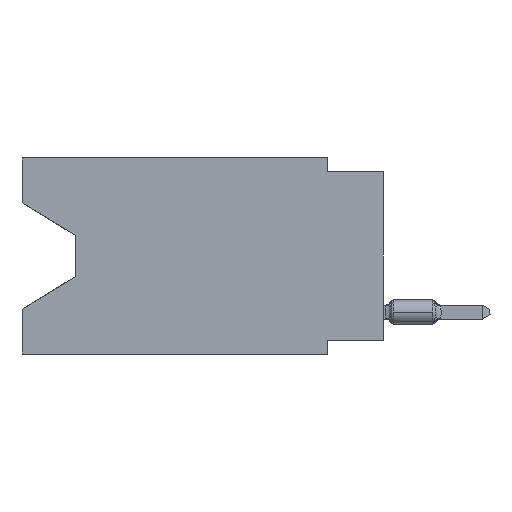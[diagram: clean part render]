
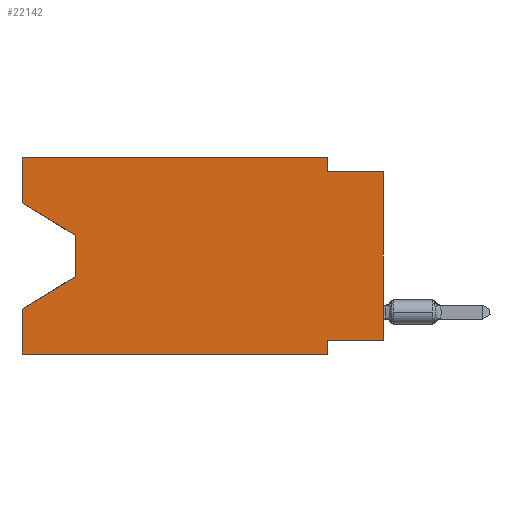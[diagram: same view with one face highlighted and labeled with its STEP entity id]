
A CAD part, left-side view. The second image highlights one B-rep face of the part: STEP entity #22142.
In plain terms, the highlighted planar face has unit normal (-1, 0, 0).
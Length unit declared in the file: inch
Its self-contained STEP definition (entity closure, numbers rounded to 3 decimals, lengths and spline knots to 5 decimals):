
#1131 = VECTOR ( 'NONE', #43221, 39.37008 ) ;
#1315 = VECTOR ( 'NONE', #15655, 39.37008 ) ;
#1429 = VECTOR ( 'NONE', #44214, 39.37008 ) ;
#1787 = EDGE_CURVE ( 'NONE', #48189, #27708, #22861, .T. ) ;
#2738 = CARTESIAN_POINT ( 'NONE',  ( 0., 0.645, 0. ) ) ;
#2757 = DIRECTION ( 'NONE',  ( 1., 0., 0. ) ) ;
#2975 = LINE ( 'NONE', #22295, #7752 ) ;
#3117 = VERTEX_POINT ( 'NONE', #30877 ) ;
#3692 = CARTESIAN_POINT ( 'NONE',  ( 0., 0.1, -0.35 ) ) ;
#3743 = LINE ( 'NONE', #29391, #39164 ) ;
#4198 = EDGE_CURVE ( 'NONE', #3117, #31693, #40388, .T. ) ;
#4311 = ORIENTED_EDGE ( 'NONE', *, *, #17514, .F. ) ;
#4424 = CARTESIAN_POINT ( 'NONE',  ( 0., 0.1, 0. ) ) ;
#4517 = DIRECTION ( 'NONE',  ( 0., 1., 0. ) ) ;
#4624 = CARTESIAN_POINT ( 'NONE',  ( 0., 0.1, 0. ) ) ;
#4648 = CARTESIAN_POINT ( 'NONE',  ( 0., 0.55, -0.138 ) ) ;
#4979 = ORIENTED_EDGE ( 'NONE', *, *, #4198, .F. ) ;
#5315 = CARTESIAN_POINT ( 'NONE',  ( 0., 0.1, -0.325 ) ) ;
#5489 = CARTESIAN_POINT ( 'NONE',  ( 0., 0., 0. ) ) ;
#5548 = CARTESIAN_POINT ( 'NONE',  ( 0., 0.645, -0.08025 ) ) ;
#6111 = VERTEX_POINT ( 'NONE', #2738 ) ;
#6238 = VERTEX_POINT ( 'NONE', #3692 ) ;
#6600 = VECTOR ( 'NONE', #21894, 39.37008 ) ;
#6947 = DIRECTION ( 'NONE',  ( 0., -1., 0. ) ) ;
#6990 = CARTESIAN_POINT ( 'NONE',  ( 0., 0., -0.025 ) ) ;
#7143 = DIRECTION ( 'NONE',  ( 0., 0., 1. ) ) ;
#7667 = CARTESIAN_POINT ( 'NONE',  ( 0., 0.645, 0. ) ) ;
#7752 = VECTOR ( 'NONE', #7143, 39.37008 ) ;
#8032 = ORIENTED_EDGE ( 'NONE', *, *, #1787, .F. ) ;
#8071 = EDGE_CURVE ( 'NONE', #24032, #3117, #37596, .T. ) ;
#10080 = LINE ( 'NONE', #39348, #1131 ) ;
#10835 = DIRECTION ( 'NONE',  ( 0., -1., 0. ) ) ;
#12255 = VERTEX_POINT ( 'NONE', #25113 ) ;
#13143 = ORIENTED_EDGE ( 'NONE', *, *, #36970, .T. ) ;
#13161 = EDGE_CURVE ( 'NONE', #6111, #24032, #3743, .T. ) ;
#14083 = DIRECTION ( 'NONE',  ( 0., 0., -1. ) ) ;
#14225 = ORIENTED_EDGE ( 'NONE', *, *, #33411, .F. ) ;
#14714 = VECTOR ( 'NONE', #14083, 39.37008 ) ;
#14769 = EDGE_CURVE ( 'NONE', #48069, #12255, #40587, .T. ) ;
#15655 = DIRECTION ( 'NONE',  ( 0., 0., -1. ) ) ;
#17514 = EDGE_CURVE ( 'NONE', #40342, #6111, #2975, .T. ) ;
#17635 = DIRECTION ( 'NONE',  ( 0., 0., -1. ) ) ;
#18287 = EDGE_CURVE ( 'NONE', #35943, #12255, #40585, .T. ) ;
#20772 = EDGE_CURVE ( 'NONE', #39972, #48069, #21679, .T. ) ;
#21679 = LINE ( 'NONE', #26050, #43831 ) ;
#21894 = DIRECTION ( 'NONE',  ( 0., -1., 0. ) ) ;
#22142 = ADVANCED_FACE ( 'NONE', ( #28397 ), #47104, .F. ) ;
#22156 = EDGE_CURVE ( 'NONE', #40342, #39972, #10080, .T. ) ;
#22295 = CARTESIAN_POINT ( 'NONE',  ( 0., 0.645, 0. ) ) ;
#22577 = CARTESIAN_POINT ( 'NONE',  ( 0., 0.645, -0.35 ) ) ;
#22861 = LINE ( 'NONE', #30881, #37675 ) ;
#22961 = VECTOR ( 'NONE', #6947, 39.37008 ) ;
#24032 = VERTEX_POINT ( 'NONE', #4624 ) ;
#24141 = ORIENTED_EDGE ( 'NONE', *, *, #13161, .F. ) ;
#25113 = CARTESIAN_POINT ( 'NONE',  ( 0., 0.645, -0.26975 ) ) ;
#26050 = CARTESIAN_POINT ( 'NONE',  ( 0., 0.55, -0.138 ) ) ;
#26614 = CARTESIAN_POINT ( 'NONE',  ( 0., 0.645, -0.35 ) ) ;
#27708 = VERTEX_POINT ( 'NONE', #5315 ) ;
#27843 = ORIENTED_EDGE ( 'NONE', *, *, #8071, .F. ) ;
#28397 = FACE_OUTER_BOUND ( 'NONE', #30882, .T. ) ;
#28431 = ORIENTED_EDGE ( 'NONE', *, *, #22156, .T. ) ;
#29391 = CARTESIAN_POINT ( 'NONE',  ( 0., 0.645, 0. ) ) ;
#29712 = DIRECTION ( 'NONE',  ( 0., 0., -1. ) ) ;
#30877 = CARTESIAN_POINT ( 'NONE',  ( 0., 0.1, -0.025 ) ) ;
#30881 = CARTESIAN_POINT ( 'NONE',  ( 0., 0., -0.325 ) ) ;
#30882 = EDGE_LOOP ( 'NONE', ( #28431, #31385, #42824, #48009, #41137, #14225, #8032, #13143, #4979, #27843, #24141, #4311 ) ) ;
#31385 = ORIENTED_EDGE ( 'NONE', *, *, #20772, .T. ) ;
#31693 = VERTEX_POINT ( 'NONE', #47474 ) ;
#32370 = LINE ( 'NONE', #40167, #14714 ) ;
#32542 = DIRECTION ( 'NONE',  ( 0., 0.855, -0.519 ) ) ;
#33049 = LINE ( 'NONE', #22577, #22961 ) ;
#33411 = EDGE_CURVE ( 'NONE', #27708, #6238, #32370, .T. ) ;
#34614 = CARTESIAN_POINT ( 'NONE',  ( 0., 0.55, -0.212 ) ) ;
#35943 = VERTEX_POINT ( 'NONE', #26614 ) ;
#36404 = CARTESIAN_POINT ( 'NONE',  ( 0., 0.645, 0. ) ) ;
#36948 = AXIS2_PLACEMENT_3D ( 'NONE', #36404, #2757, #17635 ) ;
#36970 = EDGE_CURVE ( 'NONE', #48189, #31693, #46897, .T. ) ;
#37596 = LINE ( 'NONE', #4424, #1315 ) ;
#37675 = VECTOR ( 'NONE', #4517, 39.37008 ) ;
#38664 = DIRECTION ( 'NONE',  ( 0., 0., 1. ) ) ;
#39164 = VECTOR ( 'NONE', #10835, 39.37008 ) ;
#39348 = CARTESIAN_POINT ( 'NONE',  ( 0., 0.645, -0.08025 ) ) ;
#39953 = VECTOR ( 'NONE', #32542, 39.37008 ) ;
#39972 = VERTEX_POINT ( 'NONE', #4648 ) ;
#40167 = CARTESIAN_POINT ( 'NONE',  ( 0., 0.1, -0.35 ) ) ;
#40342 = VERTEX_POINT ( 'NONE', #5548 ) ;
#40388 = LINE ( 'NONE', #6990, #6600 ) ;
#40585 = LINE ( 'NONE', #7667, #1429 ) ;
#40587 = LINE ( 'NONE', #48104, #39953 ) ;
#40962 = EDGE_CURVE ( 'NONE', #35943, #6238, #33049, .T. ) ;
#41137 = ORIENTED_EDGE ( 'NONE', *, *, #40962, .T. ) ;
#42824 = ORIENTED_EDGE ( 'NONE', *, *, #14769, .T. ) ;
#43221 = DIRECTION ( 'NONE',  ( 0., -0.855, -0.519 ) ) ;
#43831 = VECTOR ( 'NONE', #29712, 39.37008 ) ;
#44214 = DIRECTION ( 'NONE',  ( 0., 0., 1. ) ) ;
#45783 = CARTESIAN_POINT ( 'NONE',  ( 0., 0., -0.325 ) ) ;
#46736 = VECTOR ( 'NONE', #38664, 39.37008 ) ;
#46897 = LINE ( 'NONE', #5489, #46736 ) ;
#47104 = PLANE ( 'NONE',  #36948 ) ;
#47474 = CARTESIAN_POINT ( 'NONE',  ( 0., 0., -0.025 ) ) ;
#48009 = ORIENTED_EDGE ( 'NONE', *, *, #18287, .F. ) ;
#48069 = VERTEX_POINT ( 'NONE', #34614 ) ;
#48104 = CARTESIAN_POINT ( 'NONE',  ( 0., 0.55, -0.212 ) ) ;
#48189 = VERTEX_POINT ( 'NONE', #45783 ) ;
